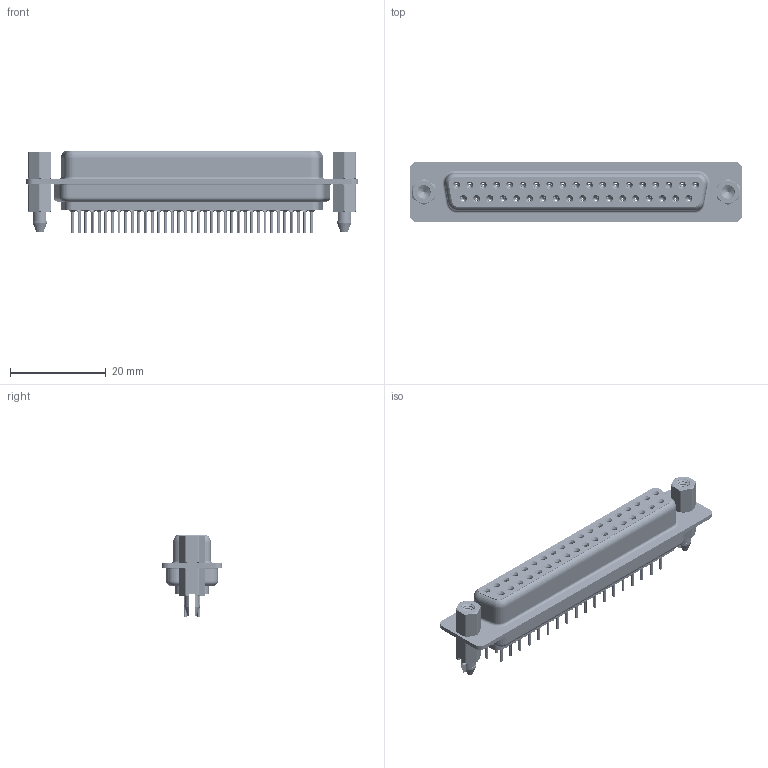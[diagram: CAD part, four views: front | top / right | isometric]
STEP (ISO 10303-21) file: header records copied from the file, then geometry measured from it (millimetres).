
FILE_DESCRIPTION (( 'STEP AP203' ), '1' );
FILE_NAME ('628-037-220-047.STEP', '2020-07-14T16:40:22', ( '' ), ( '' ), 'SwSTEP 2.0', 'SolidWorks 2020', '' );
FILE_SCHEMA (( 'CONFIG_CONTROL_DESIGN' ));
Length unit declared in the file: millimetre
Products named in the file (8): 628 Contact Row 1_20L; 628 Housing_37 LP; 628 4-40 Threaded Boardlock_LP; 628 Shell Front_37 Contacts; 628-037-220-047; 628 4-40 Hex Standoff; 628 Shell Rear_37 Contacts; 628 Contact Row 2_20L
Assembly tree (44 placements, depth 2):
  628-037-220-047
    628 Housing_37 LP
    628 Shell Front_37 Contacts
    628 Shell Rear_37 Contacts
    628 Contact Row 1_20L  x19
    628 Contact Row 2_20L  x18
    628 4-40 Hex Standoff  x2
    628 4-40 Threaded Boardlock_LP  x2
Bounding box: 69.3 x 12.6 x 17.3 mm (x, y, z)
Volume: 5706.4 mm3; surface area: 13719.4 mm2
Topology: 44 solids, 44 shells, 5178 faces, 13253 edges, 8246 vertices
Faces by surface type: cylinder 1462, plane 1268, torus 1025, bspline 758, cone 665
Entity records: 38586 total; most frequent: CARTESIAN_POINT 12036, DIRECTION 5413, ORIENTED_EDGE 5020, EDGE_CURVE 2510, AXIS2_PLACEMENT_3D 2262, VERTEX_POINT 1594, EDGE_LOOP 1260, CIRCLE 1213
